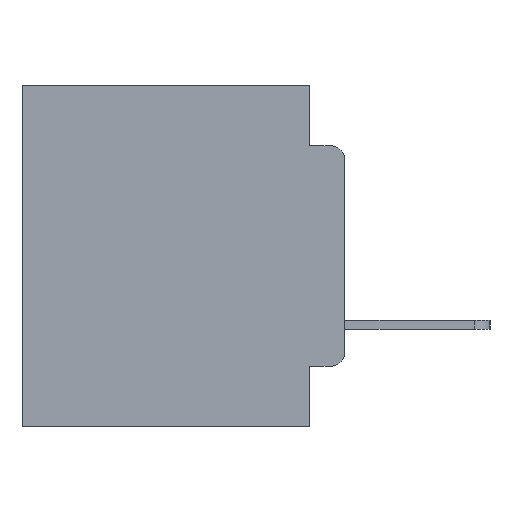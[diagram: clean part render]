
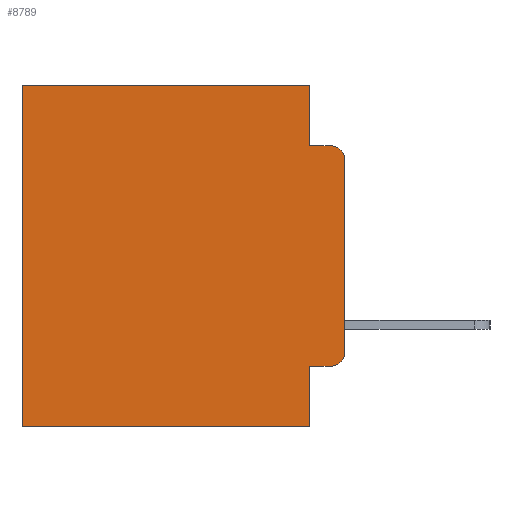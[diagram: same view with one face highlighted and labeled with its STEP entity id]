
A CAD part, left-side view. The second image highlights one B-rep face of the part: STEP entity #8789.
In plain terms, the highlighted planar face has unit normal (-1, 0, 0).
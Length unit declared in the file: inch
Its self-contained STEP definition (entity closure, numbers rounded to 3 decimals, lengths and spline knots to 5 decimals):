
#322 = EDGE_CURVE ( 'NONE', #18728, #1308, #1166, .T. ) ;
#582 = VERTEX_POINT ( 'NONE', #17711 ) ;
#1166 = LINE ( 'NONE', #14920, #12243 ) ;
#1308 = VERTEX_POINT ( 'NONE', #25006 ) ;
#1454 = EDGE_CURVE ( 'NONE', #14846, #18622, #25785, .T. ) ;
#1500 = LINE ( 'NONE', #5582, #18997 ) ;
#1574 = CARTESIAN_POINT ( 'NONE',  ( 0.298, 0.051, -0.0885 ) ) ;
#1785 = LINE ( 'NONE', #24587, #7066 ) ;
#1847 = EDGE_CURVE ( 'NONE', #17966, #22657, #1785, .T. ) ;
#1922 = CARTESIAN_POINT ( 'NONE',  ( 0.298, 0., 0. ) ) ;
#2002 = CARTESIAN_POINT ( 'NONE',  ( 0.298, 0.02, -0.1085 ) ) ;
#2493 = VECTOR ( 'NONE', #9936, 39.37008 ) ;
#3130 = CARTESIAN_POINT ( 'NONE',  ( 0.298, 0.051, 0. ) ) ;
#3890 = CARTESIAN_POINT ( 'NONE',  ( 0.298, 0.473, 0. ) ) ;
#3969 = CARTESIAN_POINT ( 'NONE',  ( 0.298, 0.02, -0.3915 ) ) ;
#4040 = EDGE_CURVE ( 'NONE', #20306, #18622, #12845, .T. ) ;
#4330 = DIRECTION ( 'NONE',  ( 0., 0., -1. ) ) ;
#4357 = DIRECTION ( 'NONE',  ( 0., 0., -1. ) ) ;
#5104 = AXIS2_PLACEMENT_3D ( 'NONE', #3969, #19180, #6250 ) ;
#5122 = EDGE_CURVE ( 'NONE', #15648, #18651, #19894, .T. ) ;
#5516 = EDGE_CURVE ( 'NONE', #17966, #20306, #23292, .T. ) ;
#5582 = CARTESIAN_POINT ( 'NONE',  ( 0.298, 0., 0. ) ) ;
#5629 = ORIENTED_EDGE ( 'NONE', *, *, #19801, .T. ) ;
#5753 = AXIS2_PLACEMENT_3D ( 'NONE', #1922, #17407, #4357 ) ;
#6250 = DIRECTION ( 'NONE',  ( 0., 0., -1. ) ) ;
#6595 = ORIENTED_EDGE ( 'NONE', *, *, #25875, .F. ) ;
#6849 = CARTESIAN_POINT ( 'NONE',  ( 0.298, 0.051, -0.0885 ) ) ;
#7027 = CARTESIAN_POINT ( 'NONE',  ( 0.298, 0., -0.1085 ) ) ;
#7040 = AXIS2_PLACEMENT_3D ( 'NONE', #2002, #17380, #4330 ) ;
#7066 = VECTOR ( 'NONE', #17543, 39.37008 ) ;
#8119 = CARTESIAN_POINT ( 'NONE',  ( 0.298, 0.02, -0.4115 ) ) ;
#8614 = CARTESIAN_POINT ( 'NONE',  ( 0.298, 0.051, 0. ) ) ;
#8789 = ADVANCED_FACE ( 'NONE', ( #22189 ), #10772, .F. ) ;
#9277 = ORIENTED_EDGE ( 'NONE', *, *, #1454, .T. ) ;
#9488 = VECTOR ( 'NONE', #16985, 39.37008 ) ;
#9936 = DIRECTION ( 'NONE',  ( 0., 0., -1. ) ) ;
#10772 = PLANE ( 'NONE',  #5753 ) ;
#11066 = CARTESIAN_POINT ( 'NONE',  ( 0.298, 0.473, -0.5 ) ) ;
#11721 = EDGE_CURVE ( 'NONE', #15648, #14846, #1500, .T. ) ;
#12243 = VECTOR ( 'NONE', #22955, 39.37008 ) ;
#12845 = LINE ( 'NONE', #22854, #17983 ) ;
#14055 = ORIENTED_EDGE ( 'NONE', *, *, #322, .F. ) ;
#14374 = CARTESIAN_POINT ( 'NONE',  ( 0.298, 0.473, 0. ) ) ;
#14846 = VERTEX_POINT ( 'NONE', #3890 ) ;
#14920 = CARTESIAN_POINT ( 'NONE',  ( 0.298, 0., 0. ) ) ;
#15111 = ORIENTED_EDGE ( 'NONE', *, *, #4040, .F. ) ;
#15332 = LINE ( 'NONE', #1574, #9488 ) ;
#15648 = VERTEX_POINT ( 'NONE', #3130 ) ;
#16753 = CARTESIAN_POINT ( 'NONE',  ( 0.298, 0.051, 0. ) ) ;
#16925 = DIRECTION ( 'NONE',  ( 0., 0., -1. ) ) ;
#16985 = DIRECTION ( 'NONE',  ( 0., -1., 0. ) ) ;
#17148 = EDGE_CURVE ( 'NONE', #18728, #582, #24612, .T. ) ;
#17227 = DIRECTION ( 'NONE',  ( 0., 0., -1. ) ) ;
#17380 = DIRECTION ( 'NONE',  ( -1., 0., 0. ) ) ;
#17407 = DIRECTION ( 'NONE',  ( 1., 0., 0. ) ) ;
#17543 = DIRECTION ( 'NONE',  ( 0., -1., 0. ) ) ;
#17711 = CARTESIAN_POINT ( 'NONE',  ( 0.298, 0.02, -0.0885 ) ) ;
#17807 = CARTESIAN_POINT ( 'NONE',  ( 0.298, 0.051, -0.4115 ) ) ;
#17966 = VERTEX_POINT ( 'NONE', #17807 ) ;
#17983 = VECTOR ( 'NONE', #26039, 39.37008 ) ;
#18403 = CARTESIAN_POINT ( 'NONE',  ( 0.298, 0.051, -0.5 ) ) ;
#18622 = VERTEX_POINT ( 'NONE', #11066 ) ;
#18651 = VERTEX_POINT ( 'NONE', #6849 ) ;
#18728 = VERTEX_POINT ( 'NONE', #7027 ) ;
#18997 = VECTOR ( 'NONE', #20593, 39.37008 ) ;
#19180 = DIRECTION ( 'NONE',  ( -1., 0., 0. ) ) ;
#19447 = ORIENTED_EDGE ( 'NONE', *, *, #5122, .F. ) ;
#19801 = EDGE_CURVE ( 'NONE', #22657, #1308, #21369, .T. ) ;
#19894 = LINE ( 'NONE', #8614, #2493 ) ;
#20306 = VERTEX_POINT ( 'NONE', #18403 ) ;
#20557 = VECTOR ( 'NONE', #17227, 39.37008 ) ;
#20593 = DIRECTION ( 'NONE',  ( 0., 1., 0. ) ) ;
#21369 = CIRCLE ( 'NONE', #5104, 0.02 ) ;
#21639 = ORIENTED_EDGE ( 'NONE', *, *, #17148, .T. ) ;
#22189 = FACE_OUTER_BOUND ( 'NONE', #22366, .T. ) ;
#22366 = EDGE_LOOP ( 'NONE', ( #14055, #21639, #6595, #19447, #24758, #9277, #15111, #25945, #27173, #5629 ) ) ;
#22657 = VERTEX_POINT ( 'NONE', #8119 ) ;
#22666 = VECTOR ( 'NONE', #16925, 39.37008 ) ;
#22854 = CARTESIAN_POINT ( 'NONE',  ( 0.298, 0., -0.5 ) ) ;
#22955 = DIRECTION ( 'NONE',  ( 0., 0., -1. ) ) ;
#23292 = LINE ( 'NONE', #16753, #22666 ) ;
#24587 = CARTESIAN_POINT ( 'NONE',  ( 0.298, 0.051, -0.4115 ) ) ;
#24612 = CIRCLE ( 'NONE', #7040, 0.02 ) ;
#24758 = ORIENTED_EDGE ( 'NONE', *, *, #11721, .T. ) ;
#25006 = CARTESIAN_POINT ( 'NONE',  ( 0.298, 0., -0.3915 ) ) ;
#25785 = LINE ( 'NONE', #14374, #20557 ) ;
#25875 = EDGE_CURVE ( 'NONE', #18651, #582, #15332, .T. ) ;
#25945 = ORIENTED_EDGE ( 'NONE', *, *, #5516, .F. ) ;
#26039 = DIRECTION ( 'NONE',  ( 0., 1., 0. ) ) ;
#27173 = ORIENTED_EDGE ( 'NONE', *, *, #1847, .T. ) ;
